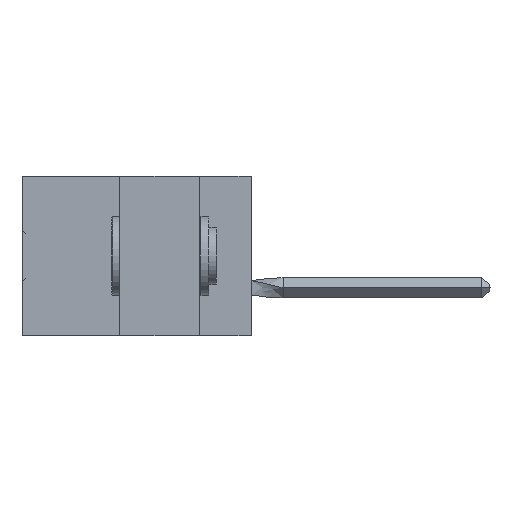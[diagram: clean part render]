
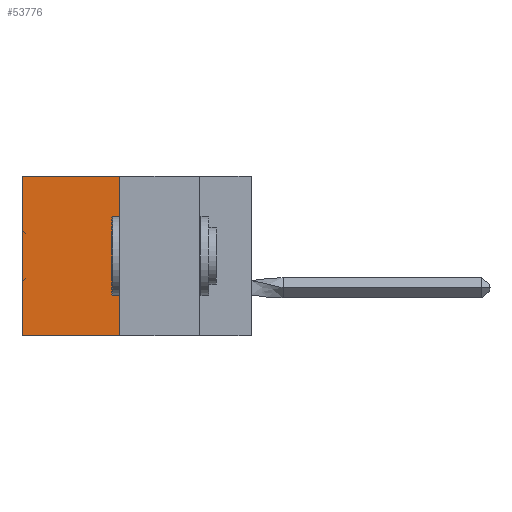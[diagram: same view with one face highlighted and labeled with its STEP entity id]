
A CAD part, left-side view. The second image highlights one B-rep face of the part: STEP entity #53776.
In plain terms, the highlighted planar face has unit normal (-1, 0, 0).
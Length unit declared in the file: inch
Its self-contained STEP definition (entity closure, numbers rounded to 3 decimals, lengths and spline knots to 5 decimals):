
#1609 = CARTESIAN_POINT ( 'NONE',  ( 0.305, 0.72, -0.5 ) ) ;
#3464 = VECTOR ( 'NONE', #16906, 39.37008 ) ;
#4974 = LINE ( 'NONE', #1609, #56894 ) ;
#7336 = PLANE ( 'NONE',  #32857 ) ;
#7939 = DIRECTION ( 'NONE',  ( 1., 0., 0. ) ) ;
#10022 = EDGE_CURVE ( 'NONE', #52035, #22200, #4974, .T. ) ;
#13317 = EDGE_CURVE ( 'NONE', #22301, #31719, #51875, .T. ) ;
#16551 = EDGE_LOOP ( 'NONE', ( #35410, #29987, #19411, #32474 ) ) ;
#16906 = DIRECTION ( 'NONE',  ( 0., 1., 0. ) ) ;
#17258 = CARTESIAN_POINT ( 'NONE',  ( 0.305, 0.413, -0.5 ) ) ;
#17568 = LINE ( 'NONE', #35219, #3464 ) ;
#18610 = CARTESIAN_POINT ( 'NONE',  ( 0.305, 0.413, 0. ) ) ;
#19411 = ORIENTED_EDGE ( 'NONE', *, *, #13317, .F. ) ;
#19637 = CARTESIAN_POINT ( 'NONE',  ( 0.305, 0.72, 0. ) ) ;
#20643 = DIRECTION ( 'NONE',  ( 0., 0., -1. ) ) ;
#20738 = VECTOR ( 'NONE', #45099, 39.37008 ) ;
#21158 = CARTESIAN_POINT ( 'NONE',  ( 0.305, 0.72, -0.5 ) ) ;
#22200 = VERTEX_POINT ( 'NONE', #21158 ) ;
#22301 = VERTEX_POINT ( 'NONE', #27760 ) ;
#22996 = DIRECTION ( 'NONE',  ( 0., 1., 0. ) ) ;
#27305 = CARTESIAN_POINT ( 'NONE',  ( 0.305, 0.413, -0.5 ) ) ;
#27760 = CARTESIAN_POINT ( 'NONE',  ( 0.305, 0.413, 0. ) ) ;
#29987 = ORIENTED_EDGE ( 'NONE', *, *, #41686, .F. ) ;
#30768 = FACE_OUTER_BOUND ( 'NONE', #16551, .T. ) ;
#31719 = VERTEX_POINT ( 'NONE', #27305 ) ;
#32474 = ORIENTED_EDGE ( 'NONE', *, *, #41324, .T. ) ;
#32857 = AXIS2_PLACEMENT_3D ( 'NONE', #17258, #7939, #35559 ) ;
#35219 = CARTESIAN_POINT ( 'NONE',  ( 0.305, 0.413, -0.5 ) ) ;
#35410 = ORIENTED_EDGE ( 'NONE', *, *, #10022, .T. ) ;
#35559 = DIRECTION ( 'NONE',  ( 0., 0., -1. ) ) ;
#41324 = EDGE_CURVE ( 'NONE', #22301, #52035, #50835, .T. ) ;
#41686 = EDGE_CURVE ( 'NONE', #31719, #22200, #17568, .T. ) ;
#45099 = DIRECTION ( 'NONE',  ( 0., 0., -1. ) ) ;
#50835 = LINE ( 'NONE', #18610, #52339 ) ;
#51875 = LINE ( 'NONE', #57649, #20738 ) ;
#52035 = VERTEX_POINT ( 'NONE', #19637 ) ;
#52339 = VECTOR ( 'NONE', #22996, 39.37008 ) ;
#53776 = ADVANCED_FACE ( 'NONE', ( #30768 ), #7336, .F. ) ;
#56894 = VECTOR ( 'NONE', #20643, 39.37008 ) ;
#57649 = CARTESIAN_POINT ( 'NONE',  ( 0.305, 0.413, -0.5 ) ) ;
